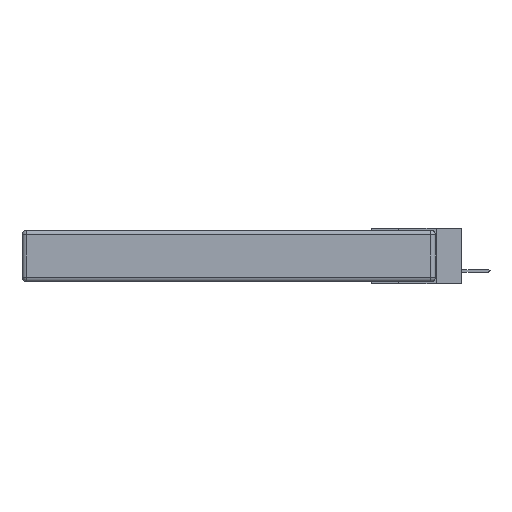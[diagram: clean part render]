
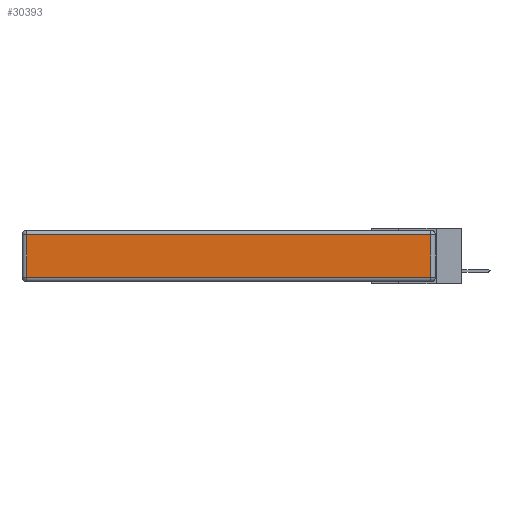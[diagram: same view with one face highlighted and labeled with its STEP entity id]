
A CAD part, left-side view. The second image highlights one B-rep face of the part: STEP entity #30393.
In plain terms, the highlighted planar face has unit normal (-1, 0, 0).
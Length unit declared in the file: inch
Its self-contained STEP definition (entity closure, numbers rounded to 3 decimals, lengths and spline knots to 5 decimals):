
#290 = ORIENTED_EDGE ( 'NONE', *, *, #2439, .T. ) ;
#350 = CARTESIAN_POINT ( 'NONE',  ( 0., 0.03, -0.03 ) ) ;
#544 = VECTOR ( 'NONE', #3948, 39.37008 ) ;
#934 = LINE ( 'NONE', #30621, #544 ) ;
#2439 = EDGE_CURVE ( 'NONE', #26452, #23908, #934, .T. ) ;
#3927 = EDGE_CURVE ( 'NONE', #23908, #4317, #31544, .T. ) ;
#3948 = DIRECTION ( 'NONE',  ( 0., -1., 0. ) ) ;
#4317 = VERTEX_POINT ( 'NONE', #350 ) ;
#4558 = LINE ( 'NONE', #18619, #26002 ) ;
#5115 = EDGE_LOOP ( 'NONE', ( #290, #12690, #29457, #12304 ) ) ;
#6423 = LINE ( 'NONE', #20945, #9365 ) ;
#7269 = DIRECTION ( 'NONE',  ( 0., 0., 1. ) ) ;
#9365 = VECTOR ( 'NONE', #16004, 39.37008 ) ;
#11853 = CARTESIAN_POINT ( 'NONE',  ( 0., 0., -0.343 ) ) ;
#12304 = ORIENTED_EDGE ( 'NONE', *, *, #25623, .T. ) ;
#12690 = ORIENTED_EDGE ( 'NONE', *, *, #3927, .T. ) ;
#13292 = VERTEX_POINT ( 'NONE', #19558 ) ;
#13335 = AXIS2_PLACEMENT_3D ( 'NONE', #11853, #17968, #7269 ) ;
#16004 = DIRECTION ( 'NONE',  ( 0., 1., 0. ) ) ;
#16971 = FACE_OUTER_BOUND ( 'NONE', #5115, .T. ) ;
#17968 = DIRECTION ( 'NONE',  ( -1., 0., 0. ) ) ;
#18206 = PLANE ( 'NONE',  #13335 ) ;
#18619 = CARTESIAN_POINT ( 'NONE',  ( 0., 2.72, -0.343 ) ) ;
#18718 = DIRECTION ( 'NONE',  ( 0., 0., 1. ) ) ;
#19558 = CARTESIAN_POINT ( 'NONE',  ( 0., 2.72, -0.03 ) ) ;
#20945 = CARTESIAN_POINT ( 'NONE',  ( 0., 2.75, -0.03 ) ) ;
#21877 = CARTESIAN_POINT ( 'NONE',  ( 0., 0.03, -0.343 ) ) ;
#22746 = VECTOR ( 'NONE', #18718, 39.37008 ) ;
#23908 = VERTEX_POINT ( 'NONE', #25964 ) ;
#25623 = EDGE_CURVE ( 'NONE', #13292, #26452, #4558, .T. ) ;
#25964 = CARTESIAN_POINT ( 'NONE',  ( 0., 0.03, -0.313 ) ) ;
#26002 = VECTOR ( 'NONE', #26553, 39.37008 ) ;
#26452 = VERTEX_POINT ( 'NONE', #31133 ) ;
#26553 = DIRECTION ( 'NONE',  ( 0., 0., -1. ) ) ;
#29457 = ORIENTED_EDGE ( 'NONE', *, *, #31010, .T. ) ;
#30393 = ADVANCED_FACE ( 'NONE', ( #16971 ), #18206, .T. ) ;
#30621 = CARTESIAN_POINT ( 'NONE',  ( 0., 0., -0.313 ) ) ;
#31010 = EDGE_CURVE ( 'NONE', #4317, #13292, #6423, .T. ) ;
#31133 = CARTESIAN_POINT ( 'NONE',  ( 0., 2.72, -0.313 ) ) ;
#31544 = LINE ( 'NONE', #21877, #22746 ) ;
